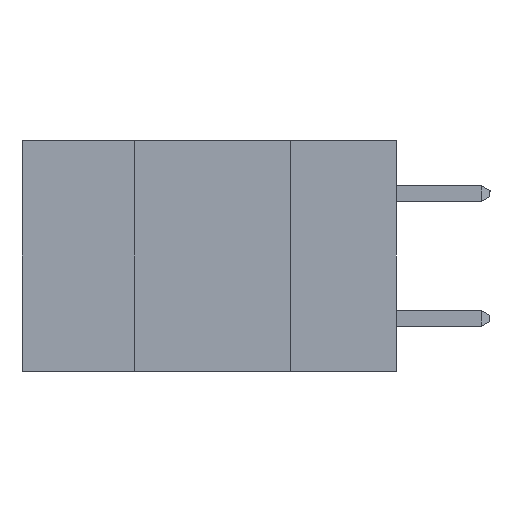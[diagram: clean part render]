
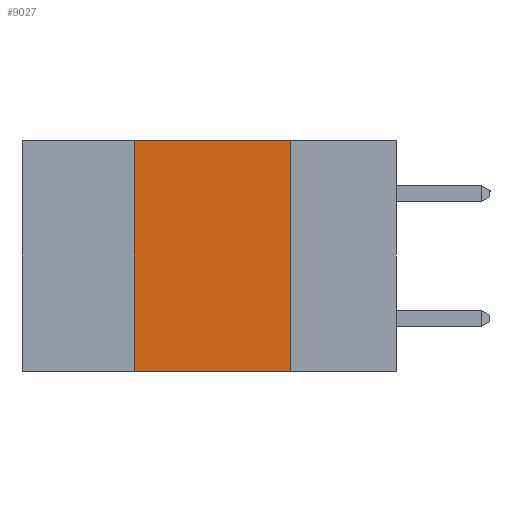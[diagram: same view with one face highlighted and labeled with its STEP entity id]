
A CAD part, left-side view. The second image highlights one B-rep face of the part: STEP entity #9027.
In plain terms, the highlighted planar face has unit normal (-1, 0, 0).
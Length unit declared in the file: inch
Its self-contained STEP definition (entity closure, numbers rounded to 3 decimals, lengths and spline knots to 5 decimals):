
#73 = DIRECTION ( 'NONE',  ( 0., 0., -1. ) ) ;
#437 = DIRECTION ( 'NONE',  ( 0., 0., 1. ) ) ;
#533 = LINE ( 'NONE', #7929, #3339 ) ;
#618 = VECTOR ( 'NONE', #1724, 39.37008 ) ;
#1269 = ORIENTED_EDGE ( 'NONE', *, *, #10352, .F. ) ;
#1297 = EDGE_CURVE ( 'NONE', #2365, #6118, #3342, .T. ) ;
#1598 = CARTESIAN_POINT ( 'NONE',  ( 0., 0.6, 0. ) ) ;
#1724 = DIRECTION ( 'NONE',  ( 0., -1., 0. ) ) ;
#2227 = CARTESIAN_POINT ( 'NONE',  ( 0., 0.42, -0.37 ) ) ;
#2365 = VERTEX_POINT ( 'NONE', #4313 ) ;
#2375 = VERTEX_POINT ( 'NONE', #5085 ) ;
#2381 = EDGE_LOOP ( 'NONE', ( #5259, #1269, #2738, #8382 ) ) ;
#2572 = DIRECTION ( 'NONE',  ( 1., 0., 0. ) ) ;
#2738 = ORIENTED_EDGE ( 'NONE', *, *, #4860, .F. ) ;
#2978 = EDGE_CURVE ( 'NONE', #2375, #6118, #533, .T. ) ;
#3339 = VECTOR ( 'NONE', #6136, 39.37008 ) ;
#3342 = LINE ( 'NONE', #9175, #618 ) ;
#4036 = FACE_OUTER_BOUND ( 'NONE', #2381, .T. ) ;
#4313 = CARTESIAN_POINT ( 'NONE',  ( 0., 0.42, -0.37 ) ) ;
#4860 = EDGE_CURVE ( 'NONE', #2365, #8930, #5442, .T. ) ;
#5085 = CARTESIAN_POINT ( 'NONE',  ( 0., 0.17, 0. ) ) ;
#5180 = VECTOR ( 'NONE', #437, 39.37008 ) ;
#5259 = ORIENTED_EDGE ( 'NONE', *, *, #2978, .F. ) ;
#5442 = LINE ( 'NONE', #2227, #5180 ) ;
#6118 = VERTEX_POINT ( 'NONE', #9377 ) ;
#6136 = DIRECTION ( 'NONE',  ( 0., 0., -1. ) ) ;
#6499 = LINE ( 'NONE', #9767, #7845 ) ;
#7198 = CARTESIAN_POINT ( 'NONE',  ( 0., 0.42, 0. ) ) ;
#7362 = PLANE ( 'NONE',  #7642 ) ;
#7642 = AXIS2_PLACEMENT_3D ( 'NONE', #1598, #2572, #73 ) ;
#7845 = VECTOR ( 'NONE', #10699, 39.37008 ) ;
#7929 = CARTESIAN_POINT ( 'NONE',  ( 0., 0.17, -0.37 ) ) ;
#8382 = ORIENTED_EDGE ( 'NONE', *, *, #1297, .T. ) ;
#8930 = VERTEX_POINT ( 'NONE', #7198 ) ;
#9027 = ADVANCED_FACE ( 'NONE', ( #4036 ), #7362, .F. ) ;
#9175 = CARTESIAN_POINT ( 'NONE',  ( 0., 0.6, -0.37 ) ) ;
#9377 = CARTESIAN_POINT ( 'NONE',  ( 0., 0.17, -0.37 ) ) ;
#9767 = CARTESIAN_POINT ( 'NONE',  ( 0., 0.6, 0. ) ) ;
#10352 = EDGE_CURVE ( 'NONE', #8930, #2375, #6499, .T. ) ;
#10699 = DIRECTION ( 'NONE',  ( 0., -1., 0. ) ) ;
